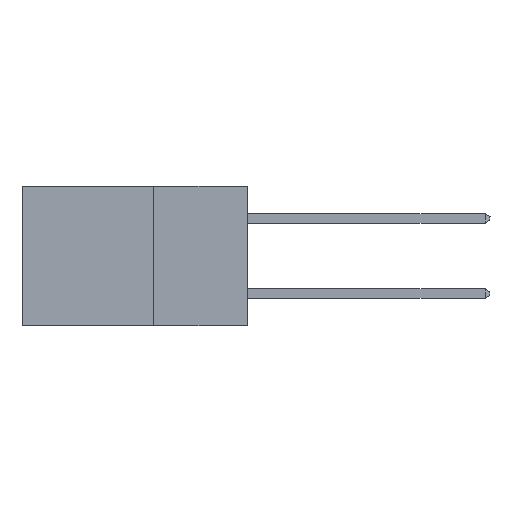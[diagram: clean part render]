
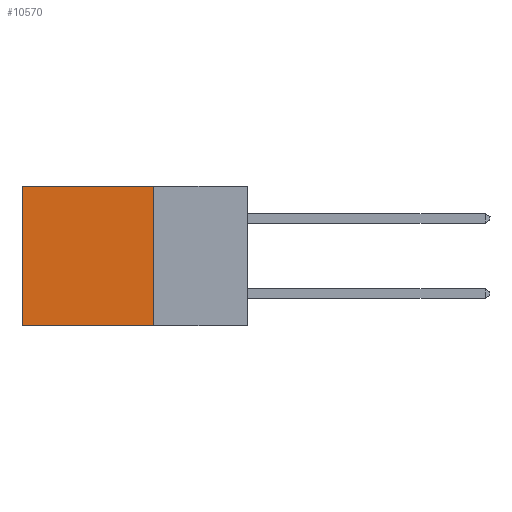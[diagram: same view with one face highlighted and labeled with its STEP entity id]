
A CAD part, left-side view. The second image highlights one B-rep face of the part: STEP entity #10570.
In plain terms, the highlighted planar face has unit normal (-1, 0, 0).
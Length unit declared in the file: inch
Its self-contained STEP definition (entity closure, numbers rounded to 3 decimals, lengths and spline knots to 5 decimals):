
#105 = CARTESIAN_POINT ( 'NONE',  ( 0.2615, 0.25, 0. ) ) ;
#677 = VECTOR ( 'NONE', #8952, 39.37008 ) ;
#1010 = DIRECTION ( 'NONE',  ( 0., 0., -1. ) ) ;
#1271 = LINE ( 'NONE', #5957, #8953 ) ;
#1753 = DIRECTION ( 'NONE',  ( 0., 0., -1. ) ) ;
#1904 = CARTESIAN_POINT ( 'NONE',  ( 0.2615, 0.6, 0. ) ) ;
#1996 = DIRECTION ( 'NONE',  ( 1., 0., 0. ) ) ;
#2595 = EDGE_LOOP ( 'NONE', ( #10181, #8211, #11807, #10134 ) ) ;
#2650 = CARTESIAN_POINT ( 'NONE',  ( 0.2615, 0.25, -0.37 ) ) ;
#2954 = PLANE ( 'NONE',  #3381 ) ;
#3013 = FACE_OUTER_BOUND ( 'NONE', #2595, .T. ) ;
#3250 = CARTESIAN_POINT ( 'NONE',  ( 0.2615, 0.6, -0.37 ) ) ;
#3381 = AXIS2_PLACEMENT_3D ( 'NONE', #7702, #1996, #1753 ) ;
#5048 = CARTESIAN_POINT ( 'NONE',  ( 0.2615, 0.25, 0. ) ) ;
#5356 = VECTOR ( 'NONE', #7931, 39.37008 ) ;
#5761 = VERTEX_POINT ( 'NONE', #5048 ) ;
#5898 = CARTESIAN_POINT ( 'NONE',  ( 0.2615, 0.6, -0.37 ) ) ;
#5957 = CARTESIAN_POINT ( 'NONE',  ( 0.2615, 0.25, -0.37 ) ) ;
#7023 = EDGE_CURVE ( 'NONE', #5761, #11393, #8925, .T. ) ;
#7508 = VECTOR ( 'NONE', #1010, 39.37008 ) ;
#7702 = CARTESIAN_POINT ( 'NONE',  ( 0.2615, 0.25, -0.37 ) ) ;
#7931 = DIRECTION ( 'NONE',  ( 0., 1., 0. ) ) ;
#8211 = ORIENTED_EDGE ( 'NONE', *, *, #9354, .F. ) ;
#8619 = LINE ( 'NONE', #2650, #7508 ) ;
#8925 = LINE ( 'NONE', #105, #5356 ) ;
#8952 = DIRECTION ( 'NONE',  ( 0., 0., -1. ) ) ;
#8953 = VECTOR ( 'NONE', #9000, 39.37008 ) ;
#8967 = EDGE_CURVE ( 'NONE', #11393, #10544, #12055, .T. ) ;
#9000 = DIRECTION ( 'NONE',  ( 0., 1., 0. ) ) ;
#9354 = EDGE_CURVE ( 'NONE', #10811, #10544, #1271, .T. ) ;
#10134 = ORIENTED_EDGE ( 'NONE', *, *, #7023, .T. ) ;
#10181 = ORIENTED_EDGE ( 'NONE', *, *, #8967, .T. ) ;
#10544 = VERTEX_POINT ( 'NONE', #5898 ) ;
#10570 = ADVANCED_FACE ( 'NONE', ( #3013 ), #2954, .F. ) ;
#10811 = VERTEX_POINT ( 'NONE', #12444 ) ;
#11393 = VERTEX_POINT ( 'NONE', #1904 ) ;
#11807 = ORIENTED_EDGE ( 'NONE', *, *, #12399, .F. ) ;
#12055 = LINE ( 'NONE', #3250, #677 ) ;
#12399 = EDGE_CURVE ( 'NONE', #5761, #10811, #8619, .T. ) ;
#12444 = CARTESIAN_POINT ( 'NONE',  ( 0.2615, 0.25, -0.37 ) ) ;
